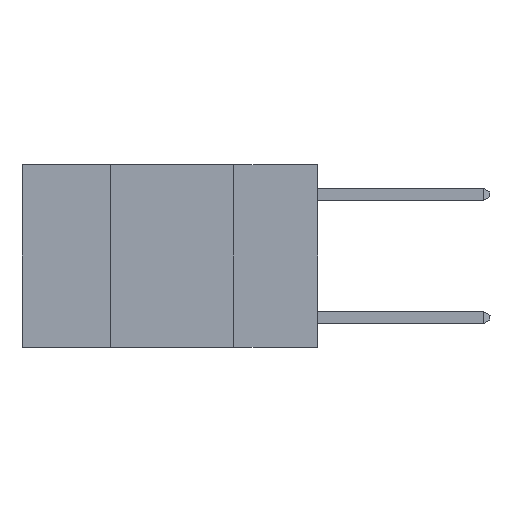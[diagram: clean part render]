
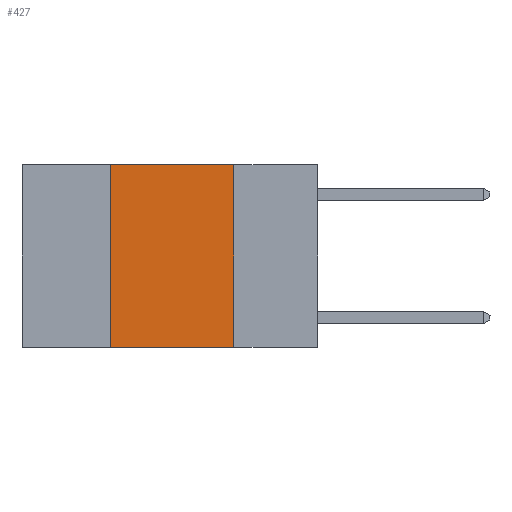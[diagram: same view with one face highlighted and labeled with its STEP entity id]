
A CAD part, left-side view. The second image highlights one B-rep face of the part: STEP entity #427.
In plain terms, the highlighted planar face has unit normal (-1, 0, 0).
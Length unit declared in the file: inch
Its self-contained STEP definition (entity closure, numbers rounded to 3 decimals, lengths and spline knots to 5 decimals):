
#283 = VECTOR ( 'NONE', #2582, 39.37008 ) ;
#427 = ADVANCED_FACE ( 'NONE', ( #11362 ), #550, .F. ) ;
#495 = CARTESIAN_POINT ( 'NONE',  ( 0., 0.17, 0. ) ) ;
#550 = PLANE ( 'NONE',  #25084 ) ;
#774 = VERTEX_POINT ( 'NONE', #495 ) ;
#871 = CARTESIAN_POINT ( 'NONE',  ( 0., 0.6, 0. ) ) ;
#911 = EDGE_CURVE ( 'NONE', #774, #11740, #3418, .T. ) ;
#1075 = VERTEX_POINT ( 'NONE', #5896 ) ;
#2012 = EDGE_CURVE ( 'NONE', #12669, #774, #13854, .T. ) ;
#2152 = CARTESIAN_POINT ( 'NONE',  ( 0., 0.6, -0.37 ) ) ;
#2263 = DIRECTION ( 'NONE',  ( 0., -1., 0. ) ) ;
#2582 = DIRECTION ( 'NONE',  ( 0., -1., 0. ) ) ;
#3418 = LINE ( 'NONE', #25690, #21629 ) ;
#3692 = DIRECTION ( 'NONE',  ( 0., 0., -1. ) ) ;
#4072 = DIRECTION ( 'NONE',  ( 1., 0., 0. ) ) ;
#5896 = CARTESIAN_POINT ( 'NONE',  ( 0., 0.42, -0.37 ) ) ;
#7306 = DIRECTION ( 'NONE',  ( 0., 0., 1. ) ) ;
#7411 = EDGE_CURVE ( 'NONE', #1075, #11740, #9986, .T. ) ;
#9986 = LINE ( 'NONE', #2152, #15533 ) ;
#11243 = CARTESIAN_POINT ( 'NONE',  ( 0., 0.6, 0. ) ) ;
#11362 = FACE_OUTER_BOUND ( 'NONE', #23134, .T. ) ;
#11740 = VERTEX_POINT ( 'NONE', #27969 ) ;
#11902 = ORIENTED_EDGE ( 'NONE', *, *, #20501, .F. ) ;
#12669 = VERTEX_POINT ( 'NONE', #28840 ) ;
#13854 = LINE ( 'NONE', #11243, #283 ) ;
#15533 = VECTOR ( 'NONE', #2263, 39.37008 ) ;
#18150 = ORIENTED_EDGE ( 'NONE', *, *, #7411, .T. ) ;
#18884 = ORIENTED_EDGE ( 'NONE', *, *, #911, .F. ) ;
#20501 = EDGE_CURVE ( 'NONE', #1075, #12669, #27095, .T. ) ;
#20837 = VECTOR ( 'NONE', #7306, 39.37008 ) ;
#21629 = VECTOR ( 'NONE', #3692, 39.37008 ) ;
#23134 = EDGE_LOOP ( 'NONE', ( #18884, #25136, #11902, #18150 ) ) ;
#25084 = AXIS2_PLACEMENT_3D ( 'NONE', #871, #4072, #29262 ) ;
#25136 = ORIENTED_EDGE ( 'NONE', *, *, #2012, .F. ) ;
#25690 = CARTESIAN_POINT ( 'NONE',  ( 0., 0.17, 0. ) ) ;
#26199 = CARTESIAN_POINT ( 'NONE',  ( 0., 0.42, 0. ) ) ;
#27095 = LINE ( 'NONE', #26199, #20837 ) ;
#27969 = CARTESIAN_POINT ( 'NONE',  ( 0., 0.17, -0.37 ) ) ;
#28840 = CARTESIAN_POINT ( 'NONE',  ( 0., 0.42, 0. ) ) ;
#29262 = DIRECTION ( 'NONE',  ( 0., 0., -1. ) ) ;
